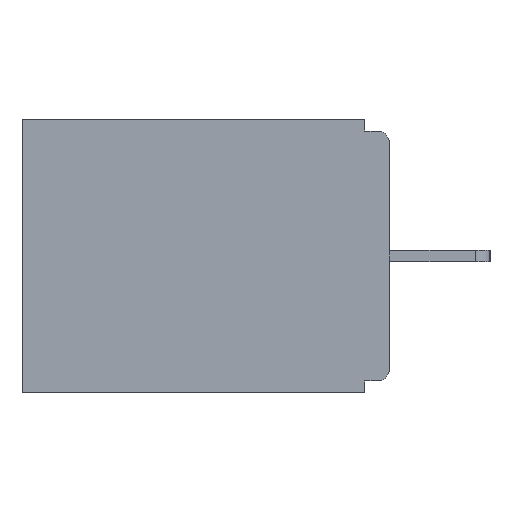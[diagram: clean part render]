
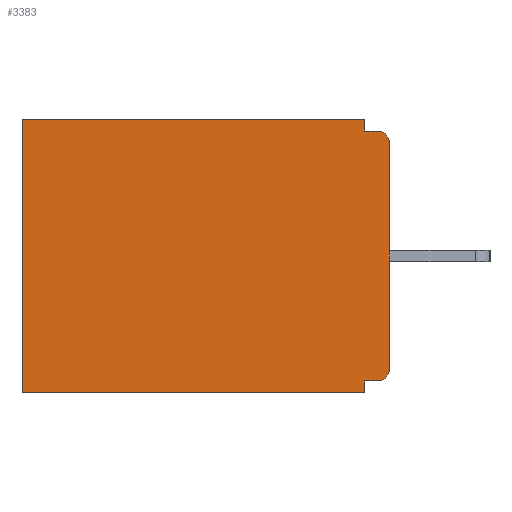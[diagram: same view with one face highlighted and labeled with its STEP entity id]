
A CAD part, left-side view. The second image highlights one B-rep face of the part: STEP entity #3383.
In plain terms, the highlighted planar face has unit normal (-1, 0, 0).
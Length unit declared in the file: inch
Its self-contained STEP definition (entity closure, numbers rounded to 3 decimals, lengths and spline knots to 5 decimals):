
#24 = DIRECTION ( 'NONE',  ( -1., 0., 0. ) ) ;
#274 = ORIENTED_EDGE ( 'NONE', *, *, #6410, .T. ) ;
#683 = AXIS2_PLACEMENT_3D ( 'NONE', #5917, #24, #6816 ) ;
#809 = VECTOR ( 'NONE', #8003, 39.37008 ) ;
#876 = DIRECTION ( 'NONE',  ( 0., 1., 0. ) ) ;
#958 = ORIENTED_EDGE ( 'NONE', *, *, #3214, .F. ) ;
#1202 = VERTEX_POINT ( 'NONE', #2824 ) ;
#1221 = EDGE_CURVE ( 'NONE', #1202, #1427, #5957, .T. ) ;
#1308 = CIRCLE ( 'NONE', #10191, 0.015 ) ;
#1427 = VERTEX_POINT ( 'NONE', #2653 ) ;
#1443 = VERTEX_POINT ( 'NONE', #2657 ) ;
#1446 = EDGE_LOOP ( 'NONE', ( #10513, #4082, #11020, #274, #5809, #8118, #10140, #958, #4249, #2834 ) ) ;
#1512 = EDGE_CURVE ( 'NONE', #5450, #1867, #7371, .T. ) ;
#1576 = CARTESIAN_POINT ( 'NONE',  ( 0.298, 0.46, 0. ) ) ;
#1659 = VERTEX_POINT ( 'NONE', #8102 ) ;
#1867 = VERTEX_POINT ( 'NONE', #3731 ) ;
#1952 = DIRECTION ( 'NONE',  ( 0., 0., -1. ) ) ;
#1984 = DIRECTION ( 'NONE',  ( 0., 1., 0. ) ) ;
#2109 = CARTESIAN_POINT ( 'NONE',  ( 0.298, 0., -0.328 ) ) ;
#2593 = AXIS2_PLACEMENT_3D ( 'NONE', #10338, #5167, #5778 ) ;
#2653 = CARTESIAN_POINT ( 'NONE',  ( 0.298, 0.031, -0.343 ) ) ;
#2657 = CARTESIAN_POINT ( 'NONE',  ( 0.298, 0.031, -0.015 ) ) ;
#2749 = CARTESIAN_POINT ( 'NONE',  ( 0.298, 0., -0.343 ) ) ;
#2761 = CARTESIAN_POINT ( 'NONE',  ( 0.298, 0., -0.03 ) ) ;
#2767 = VERTEX_POINT ( 'NONE', #9682 ) ;
#2824 = CARTESIAN_POINT ( 'NONE',  ( 0.298, 0.031, -0.328 ) ) ;
#2834 = ORIENTED_EDGE ( 'NONE', *, *, #1512, .F. ) ;
#2920 = CARTESIAN_POINT ( 'NONE',  ( 0.298, 0., -0.015 ) ) ;
#3051 = EDGE_CURVE ( 'NONE', #1443, #2767, #9974, .T. ) ;
#3084 = DIRECTION ( 'NONE',  ( 0., 0., -1. ) ) ;
#3214 = EDGE_CURVE ( 'NONE', #4330, #1202, #9745, .T. ) ;
#3383 = ADVANCED_FACE ( 'NONE', ( #9379 ), #8920, .F. ) ;
#3731 = CARTESIAN_POINT ( 'NONE',  ( 0.298, 0., -0.313 ) ) ;
#3975 = CARTESIAN_POINT ( 'NONE',  ( 0.298, 0., 0. ) ) ;
#4082 = ORIENTED_EDGE ( 'NONE', *, *, #3051, .F. ) ;
#4249 = ORIENTED_EDGE ( 'NONE', *, *, #9661, .T. ) ;
#4330 = VERTEX_POINT ( 'NONE', #6906 ) ;
#4550 = CARTESIAN_POINT ( 'NONE',  ( 0.298, 0.46, 0. ) ) ;
#4772 = CARTESIAN_POINT ( 'NONE',  ( 0.298, 0.031, -0.343 ) ) ;
#4899 = LINE ( 'NONE', #1576, #10934 ) ;
#5167 = DIRECTION ( 'NONE',  ( 1., 0., 0. ) ) ;
#5450 = VERTEX_POINT ( 'NONE', #2761 ) ;
#5778 = DIRECTION ( 'NONE',  ( 0., 0., -1. ) ) ;
#5809 = ORIENTED_EDGE ( 'NONE', *, *, #8743, .T. ) ;
#5895 = VECTOR ( 'NONE', #6764, 39.37008 ) ;
#5917 = CARTESIAN_POINT ( 'NONE',  ( 0.298, 0.015, -0.03 ) ) ;
#5957 = LINE ( 'NONE', #4772, #8252 ) ;
#6380 = EDGE_CURVE ( 'NONE', #5450, #2767, #10072, .T. ) ;
#6410 = EDGE_CURVE ( 'NONE', #7919, #9147, #11450, .T. ) ;
#6415 = VECTOR ( 'NONE', #3084, 39.37008 ) ;
#6483 = EDGE_CURVE ( 'NONE', #7919, #1443, #8629, .T. ) ;
#6764 = DIRECTION ( 'NONE',  ( 0., -1., 0. ) ) ;
#6816 = DIRECTION ( 'NONE',  ( 0., 0., -1. ) ) ;
#6906 = CARTESIAN_POINT ( 'NONE',  ( 0.298, 0.015, -0.328 ) ) ;
#7239 = DIRECTION ( 'NONE',  ( 0., 0., -1. ) ) ;
#7279 = VECTOR ( 'NONE', #1984, 39.37008 ) ;
#7353 = DIRECTION ( 'NONE',  ( 0., 0., -1. ) ) ;
#7371 = LINE ( 'NONE', #11430, #809 ) ;
#7919 = VERTEX_POINT ( 'NONE', #8718 ) ;
#7974 = VECTOR ( 'NONE', #876, 39.37008 ) ;
#8003 = DIRECTION ( 'NONE',  ( 0., 0., -1. ) ) ;
#8102 = CARTESIAN_POINT ( 'NONE',  ( 0.298, 0.46, -0.343 ) ) ;
#8118 = ORIENTED_EDGE ( 'NONE', *, *, #11340, .F. ) ;
#8252 = VECTOR ( 'NONE', #1952, 39.37008 ) ;
#8452 = CARTESIAN_POINT ( 'NONE',  ( 0.298, 0.031, -0.343 ) ) ;
#8629 = LINE ( 'NONE', #8452, #6415 ) ;
#8718 = CARTESIAN_POINT ( 'NONE',  ( 0.298, 0.031, 0. ) ) ;
#8743 = EDGE_CURVE ( 'NONE', #9147, #1659, #4899, .T. ) ;
#8920 = PLANE ( 'NONE',  #2593 ) ;
#9147 = VERTEX_POINT ( 'NONE', #4550 ) ;
#9379 = FACE_OUTER_BOUND ( 'NONE', #1446, .T. ) ;
#9661 = EDGE_CURVE ( 'NONE', #4330, #1867, #1308, .T. ) ;
#9682 = CARTESIAN_POINT ( 'NONE',  ( 0.298, 0.015, -0.015 ) ) ;
#9723 = DIRECTION ( 'NONE',  ( 0., 1., 0. ) ) ;
#9745 = LINE ( 'NONE', #2109, #7974 ) ;
#9974 = LINE ( 'NONE', #2920, #5895 ) ;
#10072 = CIRCLE ( 'NONE', #683, 0.015 ) ;
#10140 = ORIENTED_EDGE ( 'NONE', *, *, #1221, .F. ) ;
#10191 = AXIS2_PLACEMENT_3D ( 'NONE', #11199, #11210, #7353 ) ;
#10338 = CARTESIAN_POINT ( 'NONE',  ( 0.298, 0., 0. ) ) ;
#10513 = ORIENTED_EDGE ( 'NONE', *, *, #6380, .T. ) ;
#10934 = VECTOR ( 'NONE', #7239, 39.37008 ) ;
#11020 = ORIENTED_EDGE ( 'NONE', *, *, #6483, .F. ) ;
#11161 = LINE ( 'NONE', #2749, #11404 ) ;
#11199 = CARTESIAN_POINT ( 'NONE',  ( 0.298, 0.015, -0.313 ) ) ;
#11210 = DIRECTION ( 'NONE',  ( -1., 0., 0. ) ) ;
#11340 = EDGE_CURVE ( 'NONE', #1427, #1659, #11161, .T. ) ;
#11404 = VECTOR ( 'NONE', #9723, 39.37008 ) ;
#11430 = CARTESIAN_POINT ( 'NONE',  ( 0.298, 0., 0. ) ) ;
#11450 = LINE ( 'NONE', #3975, #7279 ) ;
